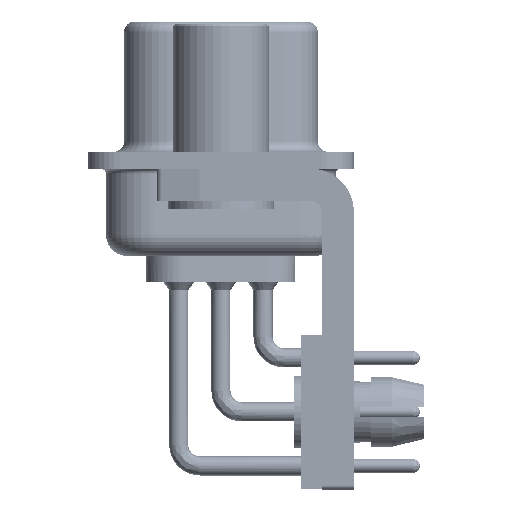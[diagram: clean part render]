
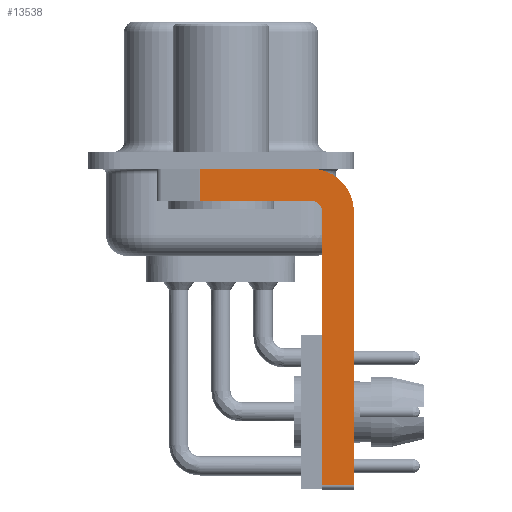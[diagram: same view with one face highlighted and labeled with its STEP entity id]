
A CAD part, left-side view. The second image highlights one B-rep face of the part: STEP entity #13538.
In plain terms, the highlighted planar face has unit normal (-1, 0, 0).
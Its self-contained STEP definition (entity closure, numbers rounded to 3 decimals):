
#762 = ORIENTED_EDGE ( 'NONE', *, *, #29807, .T. ) ;
#1988 = VECTOR ( 'NONE', #35533, 1000. ) ;
#2342 = AXIS2_PLACEMENT_3D ( 'NONE', #9559, #47385, #24676 ) ;
#3740 = LINE ( 'NONE', #25488, #42760 ) ;
#3890 = EDGE_CURVE ( 'NONE', #33704, #31019, #34120, .T. ) ;
#4600 = CARTESIAN_POINT ( 'NONE',  ( -2.9, -4.25, -2.4 ) ) ;
#5106 = VECTOR ( 'NONE', #47329, 1000. ) ;
#5357 = CARTESIAN_POINT ( 'NONE',  ( -2.9, 0.978, -1.9 ) ) ;
#5888 = CARTESIAN_POINT ( 'NONE',  ( -2.9, -4.25, -2.4 ) ) ;
#6898 = CARTESIAN_POINT ( 'NONE',  ( -2.9, -4.75, -2.4 ) ) ;
#7779 = EDGE_CURVE ( 'NONE', #18346, #26758, #3740, .T. ) ;
#7796 = VERTEX_POINT ( 'NONE', #6898 ) ;
#8404 = DIRECTION ( 'NONE',  ( 0., 0., -1. ) ) ;
#9559 = CARTESIAN_POINT ( 'NONE',  ( -2.9, -4.25, -2.4 ) ) ;
#9684 = DIRECTION ( 'NONE',  ( 0., 0., 1. ) ) ;
#10299 = CARTESIAN_POINT ( 'NONE',  ( -2.9, -6.25, -2.4 ) ) ;
#10665 = CARTESIAN_POINT ( 'NONE',  ( -2.9, -6.25, -15.25 ) ) ;
#11691 = LINE ( 'NONE', #10299, #20532 ) ;
#11721 = AXIS2_PLACEMENT_3D ( 'NONE', #5888, #32295, #9684 ) ;
#12866 = EDGE_CURVE ( 'NONE', #18346, #7796, #30818, .T. ) ;
#13538 = ADVANCED_FACE ( 'NONE', ( #46168 ), #20897, .F. ) ;
#15084 = LINE ( 'NONE', #20842, #5106 ) ;
#15467 = LINE ( 'NONE', #5357, #1988 ) ;
#18346 = VERTEX_POINT ( 'NONE', #27006 ) ;
#19662 = CARTESIAN_POINT ( 'NONE',  ( -2.9, -4.25, -1.9 ) ) ;
#20532 = VECTOR ( 'NONE', #25289, 1000. ) ;
#20769 = VECTOR ( 'NONE', #30104, 1000. ) ;
#20842 = CARTESIAN_POINT ( 'NONE',  ( -2.9, -4.25, -1.9 ) ) ;
#20897 = PLANE ( 'NONE',  #2342 ) ;
#24024 = VECTOR ( 'NONE', #41800, 1000. ) ;
#24634 = ORIENTED_EDGE ( 'NONE', *, *, #27174, .F. ) ;
#24676 = DIRECTION ( 'NONE',  ( 0., 0., -1. ) ) ;
#25289 = DIRECTION ( 'NONE',  ( 0., 0., -1. ) ) ;
#25396 = ORIENTED_EDGE ( 'NONE', *, *, #12866, .F. ) ;
#25488 = CARTESIAN_POINT ( 'NONE',  ( -2.9, -4.25, -15.25 ) ) ;
#25751 = EDGE_CURVE ( 'NONE', #35648, #26758, #11691, .T. ) ;
#26752 = ORIENTED_EDGE ( 'NONE', *, *, #25751, .F. ) ;
#26758 = VERTEX_POINT ( 'NONE', #10665 ) ;
#27006 = CARTESIAN_POINT ( 'NONE',  ( -2.9, -4.75, -15.25 ) ) ;
#27174 = EDGE_CURVE ( 'NONE', #46359, #44124, #15084, .T. ) ;
#29299 = DIRECTION ( 'NONE',  ( 0., -1., 0. ) ) ;
#29807 = EDGE_CURVE ( 'NONE', #33704, #44124, #15467, .T. ) ;
#30104 = DIRECTION ( 'NONE',  ( 0., 0., 1. ) ) ;
#30226 = ORIENTED_EDGE ( 'NONE', *, *, #41811, .F. ) ;
#30818 = LINE ( 'NONE', #41384, #20769 ) ;
#30978 = DIRECTION ( 'NONE',  ( 1., 0., 0. ) ) ;
#31019 = VERTEX_POINT ( 'NONE', #42891 ) ;
#31811 = CARTESIAN_POINT ( 'NONE',  ( -2.9, 0.978, -1.9 ) ) ;
#32295 = DIRECTION ( 'NONE',  ( -1., 0., 0. ) ) ;
#33513 = ORIENTED_EDGE ( 'NONE', *, *, #3890, .F. ) ;
#33704 = VERTEX_POINT ( 'NONE', #46960 ) ;
#34120 = LINE ( 'NONE', #43684, #24024 ) ;
#35533 = DIRECTION ( 'NONE',  ( 0., 0., -1. ) ) ;
#35648 = VERTEX_POINT ( 'NONE', #37629 ) ;
#37629 = CARTESIAN_POINT ( 'NONE',  ( -2.9, -6.25, -2.4 ) ) ;
#38015 = CIRCLE ( 'NONE', #11721, 0.5 ) ;
#39091 = ORIENTED_EDGE ( 'NONE', *, *, #7779, .T. ) ;
#41384 = CARTESIAN_POINT ( 'NONE',  ( -2.9, -4.75, -15.5 ) ) ;
#41800 = DIRECTION ( 'NONE',  ( 0., -1., 0. ) ) ;
#41811 = EDGE_CURVE ( 'NONE', #7796, #46359, #38015, .T. ) ;
#42760 = VECTOR ( 'NONE', #29299, 1000. ) ;
#42891 = CARTESIAN_POINT ( 'NONE',  ( -2.9, -4.25, -0.4 ) ) ;
#43684 = CARTESIAN_POINT ( 'NONE',  ( -2.9, 3., -0.4 ) ) ;
#44124 = VERTEX_POINT ( 'NONE', #31811 ) ;
#44551 = CIRCLE ( 'NONE', #45740, 2. ) ;
#45123 = ORIENTED_EDGE ( 'NONE', *, *, #45716, .F. ) ;
#45716 = EDGE_CURVE ( 'NONE', #31019, #35648, #44551, .T. ) ;
#45740 = AXIS2_PLACEMENT_3D ( 'NONE', #4600, #30978, #8404 ) ;
#46168 = FACE_OUTER_BOUND ( 'NONE', #47858, .T. ) ;
#46359 = VERTEX_POINT ( 'NONE', #19662 ) ;
#46960 = CARTESIAN_POINT ( 'NONE',  ( -2.9, 0.978, -0.4 ) ) ;
#47329 = DIRECTION ( 'NONE',  ( 0., 1., 0. ) ) ;
#47385 = DIRECTION ( 'NONE',  ( 1., 0., 0. ) ) ;
#47858 = EDGE_LOOP ( 'NONE', ( #33513, #762, #24634, #30226, #25396, #39091, #26752, #45123 ) ) ;
